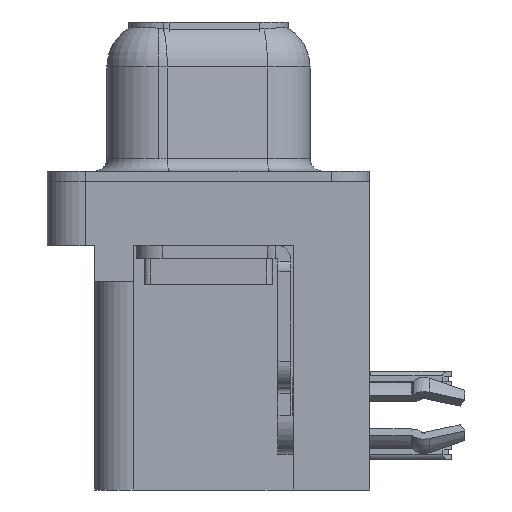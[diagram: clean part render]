
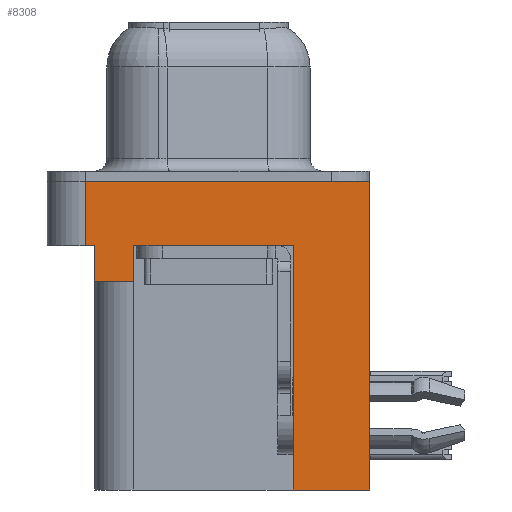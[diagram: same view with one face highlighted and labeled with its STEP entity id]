
A CAD part, left-side view. The second image highlights one B-rep face of the part: STEP entity #8308.
In plain terms, the highlighted planar face has unit normal (-1, 0, 0).
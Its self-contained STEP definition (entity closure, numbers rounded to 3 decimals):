
#17 = CARTESIAN_POINT ( 'NONE',  ( -2.935, 4.425, -3.9 ) ) ;
#183 = CARTESIAN_POINT ( 'NONE',  ( -2.935, -3.295, -12. ) ) ;
#625 = LINE ( 'NONE', #183, #6611 ) ;
#1739 = VERTEX_POINT ( 'NONE', #2178 ) ;
#2178 = CARTESIAN_POINT ( 'NONE',  ( -2.935, -3.295, -2.5 ) ) ;
#2265 = EDGE_CURVE ( 'NONE', #4416, #22480, #13091, .T. ) ;
#2327 = ORIENTED_EDGE ( 'NONE', *, *, #13041, .F. ) ;
#3511 = DIRECTION ( 'NONE',  ( 0., 0., 1. ) ) ;
#3883 = EDGE_CURVE ( 'NONE', #5726, #10269, #20467, .T. ) ;
#4025 = DIRECTION ( 'NONE',  ( 0., 1., 0. ) ) ;
#4416 = VERTEX_POINT ( 'NONE', #13983 ) ;
#4493 = EDGE_LOOP ( 'NONE', ( #25789, #5278, #17722, #24725, #13897, #24418, #16179, #8907, #2327, #9751 ) ) ;
#4501 = VERTEX_POINT ( 'NONE', #17 ) ;
#4774 = LINE ( 'NONE', #17995, #25165 ) ;
#5040 = CARTESIAN_POINT ( 'NONE',  ( -2.935, -3.295, -12. ) ) ;
#5215 = CARTESIAN_POINT ( 'NONE',  ( -2.935, -6.275, 0. ) ) ;
#5278 = ORIENTED_EDGE ( 'NONE', *, *, #13156, .F. ) ;
#5420 = VECTOR ( 'NONE', #19440, 1000. ) ;
#5726 = VERTEX_POINT ( 'NONE', #22095 ) ;
#5903 = DIRECTION ( 'NONE',  ( 0., 0., 1. ) ) ;
#6291 = VERTEX_POINT ( 'NONE', #14622 ) ;
#6611 = VECTOR ( 'NONE', #14346, 1000. ) ;
#7235 = LINE ( 'NONE', #12878, #13604 ) ;
#8050 = CARTESIAN_POINT ( 'NONE',  ( -2.935, -6.275, 0. ) ) ;
#8308 = ADVANCED_FACE ( 'NONE', ( #12173 ), #13587, .T. ) ;
#8642 = CARTESIAN_POINT ( 'NONE',  ( -2.935, 4.425, -3.9 ) ) ;
#8907 = ORIENTED_EDGE ( 'NONE', *, *, #12062, .F. ) ;
#9751 = ORIENTED_EDGE ( 'NONE', *, *, #2265, .T. ) ;
#9900 = CARTESIAN_POINT ( 'NONE',  ( -2.935, 4.425, -2.5 ) ) ;
#10269 = VERTEX_POINT ( 'NONE', #14185 ) ;
#10308 = CARTESIAN_POINT ( 'NONE',  ( -2.935, -6.275, -2.5 ) ) ;
#11629 = LINE ( 'NONE', #8642, #12944 ) ;
#11661 = DIRECTION ( 'NONE',  ( 0., 0., 1. ) ) ;
#11759 = CARTESIAN_POINT ( 'NONE',  ( -2.935, -6.275, -2.5 ) ) ;
#12062 = EDGE_CURVE ( 'NONE', #14909, #1739, #4774, .T. ) ;
#12173 = FACE_OUTER_BOUND ( 'NONE', #4493, .T. ) ;
#12262 = VECTOR ( 'NONE', #21928, 1000. ) ;
#12354 = VECTOR ( 'NONE', #23930, 1000. ) ;
#12507 = EDGE_CURVE ( 'NONE', #6291, #21332, #23234, .T. ) ;
#12878 = CARTESIAN_POINT ( 'NONE',  ( -2.935, 4.775, -2.5 ) ) ;
#12944 = VECTOR ( 'NONE', #18725, 1000. ) ;
#13041 = EDGE_CURVE ( 'NONE', #4416, #14909, #625, .T. ) ;
#13091 = LINE ( 'NONE', #10308, #22332 ) ;
#13156 = EDGE_CURVE ( 'NONE', #6291, #25507, #7235, .T. ) ;
#13587 = PLANE ( 'NONE',  #25438 ) ;
#13601 = EDGE_CURVE ( 'NONE', #4501, #21332, #11629, .T. ) ;
#13604 = VECTOR ( 'NONE', #21086, 1000. ) ;
#13897 = ORIENTED_EDGE ( 'NONE', *, *, #25665, .F. ) ;
#13983 = CARTESIAN_POINT ( 'NONE',  ( -2.935, -6.275, -12. ) ) ;
#14185 = CARTESIAN_POINT ( 'NONE',  ( -2.935, 2.895, -2.5 ) ) ;
#14346 = DIRECTION ( 'NONE',  ( 0., 1., 0. ) ) ;
#14470 = LINE ( 'NONE', #22393, #25969 ) ;
#14622 = CARTESIAN_POINT ( 'NONE',  ( -2.935, 4.775, -2.5 ) ) ;
#14909 = VERTEX_POINT ( 'NONE', #5040 ) ;
#15064 = VECTOR ( 'NONE', #11661, 1000. ) ;
#15665 = DIRECTION ( 'NONE',  ( -1., 0., 0. ) ) ;
#16179 = ORIENTED_EDGE ( 'NONE', *, *, #20816, .T. ) ;
#17224 = CARTESIAN_POINT ( 'NONE',  ( -2.935, 2.895, -3.9 ) ) ;
#17722 = ORIENTED_EDGE ( 'NONE', *, *, #12507, .T. ) ;
#17725 = LINE ( 'NONE', #25890, #12262 ) ;
#17878 = CARTESIAN_POINT ( 'NONE',  ( -2.935, 4.775, 0. ) ) ;
#17995 = CARTESIAN_POINT ( 'NONE',  ( -2.935, -3.295, -12. ) ) ;
#18725 = DIRECTION ( 'NONE',  ( 0., 0., 1. ) ) ;
#19411 = CARTESIAN_POINT ( 'NONE',  ( -2.935, -6.275, -2.5 ) ) ;
#19440 = DIRECTION ( 'NONE',  ( 0., -1., 0. ) ) ;
#20467 = LINE ( 'NONE', #17224, #15064 ) ;
#20816 = EDGE_CURVE ( 'NONE', #10269, #1739, #17725, .T. ) ;
#21086 = DIRECTION ( 'NONE',  ( 0., 0., 1. ) ) ;
#21332 = VERTEX_POINT ( 'NONE', #9900 ) ;
#21928 = DIRECTION ( 'NONE',  ( 0., -1., 0. ) ) ;
#22095 = CARTESIAN_POINT ( 'NONE',  ( -2.935, 2.895, -3.9 ) ) ;
#22332 = VECTOR ( 'NONE', #24537, 1000. ) ;
#22393 = CARTESIAN_POINT ( 'NONE',  ( -2.935, 4.425, -3.9 ) ) ;
#22480 = VERTEX_POINT ( 'NONE', #8050 ) ;
#23234 = LINE ( 'NONE', #11759, #12354 ) ;
#23430 = EDGE_CURVE ( 'NONE', #25507, #22480, #25162, .T. ) ;
#23930 = DIRECTION ( 'NONE',  ( 0., -1., 0. ) ) ;
#24418 = ORIENTED_EDGE ( 'NONE', *, *, #3883, .T. ) ;
#24537 = DIRECTION ( 'NONE',  ( 0., 0., 1. ) ) ;
#24725 = ORIENTED_EDGE ( 'NONE', *, *, #13601, .F. ) ;
#25162 = LINE ( 'NONE', #5215, #5420 ) ;
#25165 = VECTOR ( 'NONE', #5903, 1000. ) ;
#25438 = AXIS2_PLACEMENT_3D ( 'NONE', #19411, #15665, #3511 ) ;
#25507 = VERTEX_POINT ( 'NONE', #17878 ) ;
#25665 = EDGE_CURVE ( 'NONE', #5726, #4501, #14470, .T. ) ;
#25789 = ORIENTED_EDGE ( 'NONE', *, *, #23430, .F. ) ;
#25890 = CARTESIAN_POINT ( 'NONE',  ( -2.935, -6.275, -2.5 ) ) ;
#25969 = VECTOR ( 'NONE', #4025, 1000. ) ;
